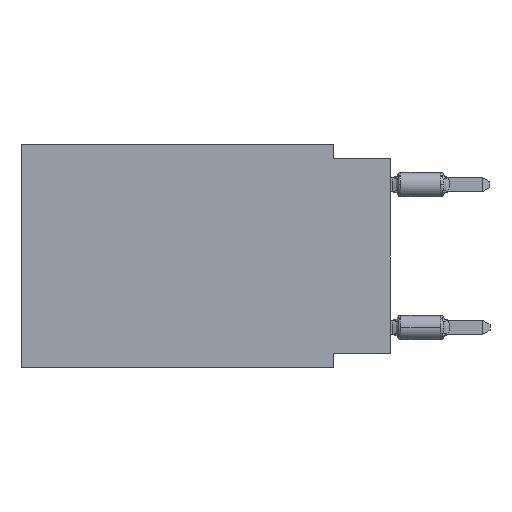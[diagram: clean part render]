
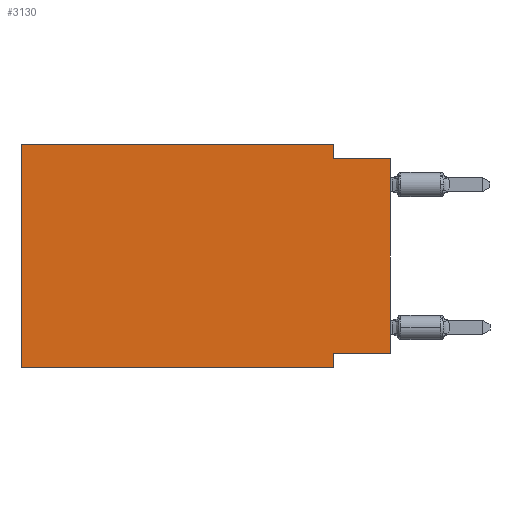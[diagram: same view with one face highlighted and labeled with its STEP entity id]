
A CAD part, left-side view. The second image highlights one B-rep face of the part: STEP entity #3130.
In plain terms, the highlighted planar face has unit normal (-1, 0, 0).
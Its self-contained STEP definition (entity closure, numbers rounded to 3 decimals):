
#622 = DIRECTION ( 'NONE',  ( 0., 0., 1. ) ) ;
#917 = CARTESIAN_POINT ( 'NONE',  ( 0., 2.54, 0. ) ) ;
#1107 = EDGE_CURVE ( 'NONE', #16499, #5445, #3801, .T. ) ;
#1825 = FACE_OUTER_BOUND ( 'NONE', #8462, .T. ) ;
#2342 = AXIS2_PLACEMENT_3D ( 'NONE', #8139, #8220, #16315 ) ;
#2762 = ORIENTED_EDGE ( 'NONE', *, *, #2874, .T. ) ;
#2796 = PLANE ( 'NONE',  #2342 ) ;
#2842 = VECTOR ( 'NONE', #13507, 1000. ) ;
#2874 = EDGE_CURVE ( 'NONE', #16499, #10823, #12651, .T. ) ;
#2911 = VECTOR ( 'NONE', #7659, 1000. ) ;
#2993 = CARTESIAN_POINT ( 'NONE',  ( 0., 2.54, -9.271 ) ) ;
#3130 = ADVANCED_FACE ( 'NONE', ( #1825 ), #2796, .F. ) ;
#3801 = LINE ( 'NONE', #17138, #15752 ) ;
#4030 = VECTOR ( 'NONE', #15399, 1000. ) ;
#4159 = EDGE_CURVE ( 'NONE', #15582, #14285, #10303, .T. ) ;
#4743 = CARTESIAN_POINT ( 'NONE',  ( 0., 0., 0. ) ) ;
#4872 = CARTESIAN_POINT ( 'NONE',  ( 0., 0., -9.271 ) ) ;
#5028 = EDGE_CURVE ( 'NONE', #5445, #14285, #10665, .T. ) ;
#5053 = VERTEX_POINT ( 'NONE', #6958 ) ;
#5220 = CARTESIAN_POINT ( 'NONE',  ( 0., 2.54, -9.906 ) ) ;
#5253 = EDGE_CURVE ( 'NONE', #15582, #10045, #11270, .T. ) ;
#5294 = ORIENTED_EDGE ( 'NONE', *, *, #4159, .T. ) ;
#5444 = CARTESIAN_POINT ( 'NONE',  ( 0., 2.54, -9.906 ) ) ;
#5445 = VERTEX_POINT ( 'NONE', #2993 ) ;
#6533 = DIRECTION ( 'NONE',  ( 0., 0., -1. ) ) ;
#6821 = CARTESIAN_POINT ( 'NONE',  ( 0., 0., -0.635 ) ) ;
#6958 = CARTESIAN_POINT ( 'NONE',  ( 0., 2.54, -0.635 ) ) ;
#7659 = DIRECTION ( 'NONE',  ( 0., -1., 0. ) ) ;
#7929 = CARTESIAN_POINT ( 'NONE',  ( 0., 2.54, 0. ) ) ;
#8139 = CARTESIAN_POINT ( 'NONE',  ( 0., 16.383, 0. ) ) ;
#8220 = DIRECTION ( 'NONE',  ( 1., 0., 0. ) ) ;
#8430 = CARTESIAN_POINT ( 'NONE',  ( 0., 16.383, 0. ) ) ;
#8462 = EDGE_LOOP ( 'NONE', ( #2762, #10821, #13428, #14211, #14320, #5294, #15275, #13126 ) ) ;
#8704 = VECTOR ( 'NONE', #6533, 1000. ) ;
#9139 = DIRECTION ( 'NONE',  ( 0., 1., 0. ) ) ;
#9379 = VECTOR ( 'NONE', #10580, 1000. ) ;
#9504 = LINE ( 'NONE', #7929, #8704 ) ;
#10045 = VERTEX_POINT ( 'NONE', #8430 ) ;
#10303 = LINE ( 'NONE', #15748, #2911 ) ;
#10580 = DIRECTION ( 'NONE',  ( 0., 0., -1. ) ) ;
#10656 = DIRECTION ( 'NONE',  ( 0., -1., 0. ) ) ;
#10665 = LINE ( 'NONE', #5220, #9379 ) ;
#10821 = ORIENTED_EDGE ( 'NONE', *, *, #14691, .F. ) ;
#10823 = VERTEX_POINT ( 'NONE', #11740 ) ;
#11188 = CARTESIAN_POINT ( 'NONE',  ( 0., 16.383, 0. ) ) ;
#11242 = CARTESIAN_POINT ( 'NONE',  ( 0., 16.383, -9.906 ) ) ;
#11270 = LINE ( 'NONE', #11188, #4030 ) ;
#11292 = EDGE_CURVE ( 'NONE', #10045, #15346, #15850, .T. ) ;
#11740 = CARTESIAN_POINT ( 'NONE',  ( 0., 0., -0.635 ) ) ;
#11781 = VECTOR ( 'NONE', #622, 1000. ) ;
#12136 = CARTESIAN_POINT ( 'NONE',  ( 0., 16.383, 0. ) ) ;
#12187 = VECTOR ( 'NONE', #10656, 1000. ) ;
#12651 = LINE ( 'NONE', #4743, #11781 ) ;
#13126 = ORIENTED_EDGE ( 'NONE', *, *, #1107, .F. ) ;
#13428 = ORIENTED_EDGE ( 'NONE', *, *, #13591, .F. ) ;
#13507 = DIRECTION ( 'NONE',  ( 0., -1., 0. ) ) ;
#13591 = EDGE_CURVE ( 'NONE', #15346, #5053, #9504, .T. ) ;
#14211 = ORIENTED_EDGE ( 'NONE', *, *, #11292, .F. ) ;
#14285 = VERTEX_POINT ( 'NONE', #5444 ) ;
#14320 = ORIENTED_EDGE ( 'NONE', *, *, #5253, .F. ) ;
#14691 = EDGE_CURVE ( 'NONE', #5053, #10823, #17195, .T. ) ;
#15275 = ORIENTED_EDGE ( 'NONE', *, *, #5028, .F. ) ;
#15346 = VERTEX_POINT ( 'NONE', #917 ) ;
#15399 = DIRECTION ( 'NONE',  ( 0., 0., 1. ) ) ;
#15582 = VERTEX_POINT ( 'NONE', #11242 ) ;
#15748 = CARTESIAN_POINT ( 'NONE',  ( 0., 16.383, -9.906 ) ) ;
#15752 = VECTOR ( 'NONE', #9139, 1000. ) ;
#15850 = LINE ( 'NONE', #12136, #12187 ) ;
#16315 = DIRECTION ( 'NONE',  ( 0., 0., -1. ) ) ;
#16499 = VERTEX_POINT ( 'NONE', #4872 ) ;
#17138 = CARTESIAN_POINT ( 'NONE',  ( 0., 0., -9.271 ) ) ;
#17195 = LINE ( 'NONE', #6821, #2842 ) ;
